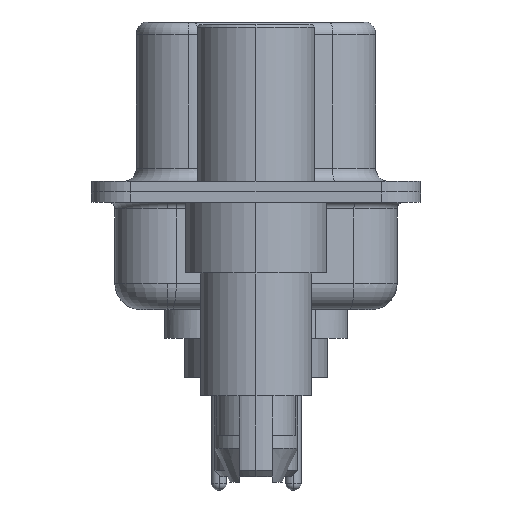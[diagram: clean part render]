
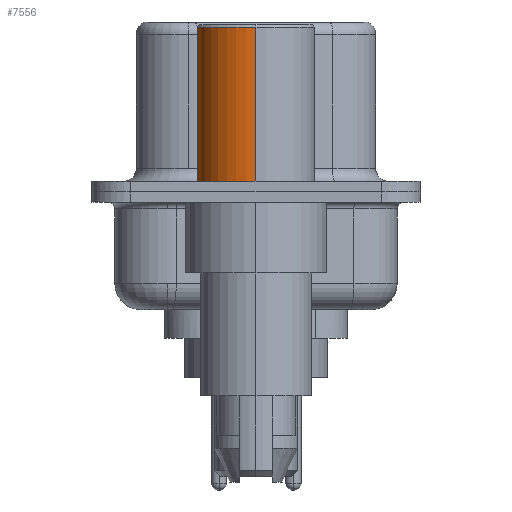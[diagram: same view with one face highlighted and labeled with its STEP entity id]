
A CAD part, left-side view. The second image highlights one B-rep face of the part: STEP entity #7556.
In plain terms, the highlighted cylindrical face has radius 2.25 mm (diameter 4.5 mm), a partial arc.
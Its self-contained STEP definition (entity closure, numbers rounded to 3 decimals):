
#15 = VECTOR ( 'NONE', #12612, 1000. ) ;
#853 = AXIS2_PLACEMENT_3D ( 'NONE', #10324, #9481, #9445 ) ;
#902 = CIRCLE ( 'NONE', #853, 2.25 ) ;
#1606 = CARTESIAN_POINT ( 'NONE',  ( -2.25, 0., 0.581 ) ) ;
#1931 = LINE ( 'NONE', #14303, #9052 ) ;
#2014 = CARTESIAN_POINT ( 'NONE',  ( 0., 0., 0.581 ) ) ;
#2092 = CARTESIAN_POINT ( 'NONE',  ( 2.25, 0., 0.4 ) ) ;
#2384 = EDGE_CURVE ( 'NONE', #13614, #3234, #902, .T. ) ;
#3234 = VERTEX_POINT ( 'NONE', #11474 ) ;
#3286 = CARTESIAN_POINT ( 'NONE',  ( 0., 0., 6.3 ) ) ;
#3335 = DIRECTION ( 'NONE',  ( 1., 0., 0. ) ) ;
#3548 = DIRECTION ( 'NONE',  ( 0., 0., 1. ) ) ;
#4651 = DIRECTION ( 'NONE',  ( 1., 0., 0. ) ) ;
#6047 = EDGE_CURVE ( 'NONE', #3234, #10989, #7627, .T. ) ;
#6893 = EDGE_LOOP ( 'NONE', ( #8629, #11200, #16982, #17283 ) ) ;
#7556 = ADVANCED_FACE ( 'NONE', ( #14079 ), #9688, .T. ) ;
#7627 = LINE ( 'NONE', #1606, #15 ) ;
#8629 = ORIENTED_EDGE ( 'NONE', *, *, #2384, .T. ) ;
#9052 = VECTOR ( 'NONE', #3548, 1000. ) ;
#9445 = DIRECTION ( 'NONE',  ( 1., 0., 0. ) ) ;
#9481 = DIRECTION ( 'NONE',  ( 0., 0., 1. ) ) ;
#9607 = CIRCLE ( 'NONE', #13536, 2.25 ) ;
#9688 = CYLINDRICAL_SURFACE ( 'NONE', #13701, 2.25 ) ;
#10059 = CARTESIAN_POINT ( 'NONE',  ( 2.25, 0., 6.3 ) ) ;
#10093 = DIRECTION ( 'NONE',  ( 0., 0., 1. ) ) ;
#10324 = CARTESIAN_POINT ( 'NONE',  ( 0., 0., 0.4 ) ) ;
#10650 = EDGE_CURVE ( 'NONE', #13614, #15092, #1931, .T. ) ;
#10981 = CARTESIAN_POINT ( 'NONE',  ( -2.25, 0., 6.3 ) ) ;
#10989 = VERTEX_POINT ( 'NONE', #10981 ) ;
#11200 = ORIENTED_EDGE ( 'NONE', *, *, #6047, .T. ) ;
#11474 = CARTESIAN_POINT ( 'NONE',  ( -2.25, 0., 0.4 ) ) ;
#12612 = DIRECTION ( 'NONE',  ( 0., 0., 1. ) ) ;
#12741 = DIRECTION ( 'NONE',  ( 0., 0., 1. ) ) ;
#13536 = AXIS2_PLACEMENT_3D ( 'NONE', #3286, #12741, #4651 ) ;
#13555 = EDGE_CURVE ( 'NONE', #15092, #10989, #9607, .T. ) ;
#13614 = VERTEX_POINT ( 'NONE', #2092 ) ;
#13701 = AXIS2_PLACEMENT_3D ( 'NONE', #2014, #10093, #3335 ) ;
#14079 = FACE_OUTER_BOUND ( 'NONE', #6893, .T. ) ;
#14303 = CARTESIAN_POINT ( 'NONE',  ( 2.25, 0., 0.581 ) ) ;
#15092 = VERTEX_POINT ( 'NONE', #10059 ) ;
#16982 = ORIENTED_EDGE ( 'NONE', *, *, #13555, .F. ) ;
#17283 = ORIENTED_EDGE ( 'NONE', *, *, #10650, .F. ) ;
